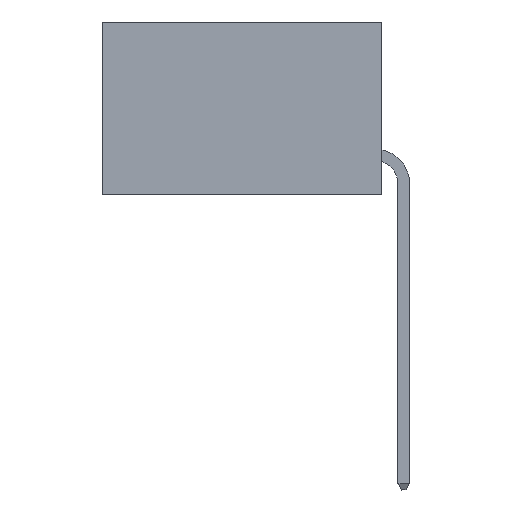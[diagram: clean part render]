
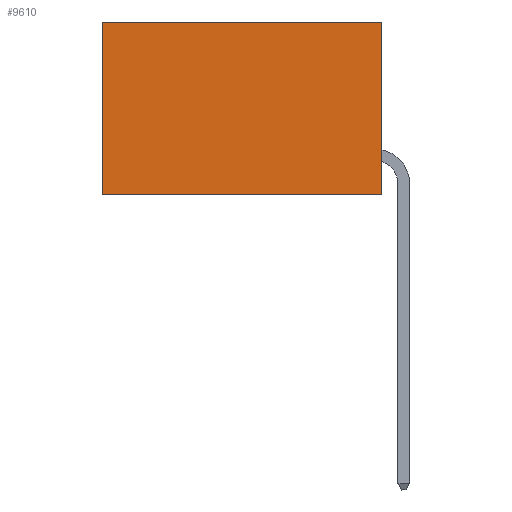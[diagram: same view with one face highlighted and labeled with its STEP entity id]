
A CAD part, left-side view. The second image highlights one B-rep face of the part: STEP entity #9610.
In plain terms, the highlighted planar face has unit normal (-1, 0, 0).
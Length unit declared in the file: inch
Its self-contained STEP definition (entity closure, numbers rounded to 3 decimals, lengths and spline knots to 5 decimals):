
#6 = EDGE_CURVE ( 'NONE', #14427, #11223, #9712, .T. ) ;
#198 = DIRECTION ( 'NONE',  ( 0., 0., -1. ) ) ;
#289 = EDGE_CURVE ( 'NONE', #11223, #3295, #1938, .T. ) ;
#1352 = VECTOR ( 'NONE', #15638, 39.37008 ) ;
#1938 = LINE ( 'NONE', #3981, #13541 ) ;
#2998 = CARTESIAN_POINT ( 'NONE',  ( 0.2875, 0., 0. ) ) ;
#3295 = VERTEX_POINT ( 'NONE', #11561 ) ;
#3981 = CARTESIAN_POINT ( 'NONE',  ( 0.2875, 0.6, 0. ) ) ;
#6026 = ORIENTED_EDGE ( 'NONE', *, *, #6596, .F. ) ;
#6596 = EDGE_CURVE ( 'NONE', #14427, #11262, #14353, .T. ) ;
#7561 = VECTOR ( 'NONE', #11308, 39.37008 ) ;
#7683 = DIRECTION ( 'NONE',  ( 1., 0., 0. ) ) ;
#8550 = AXIS2_PLACEMENT_3D ( 'NONE', #10078, #7683, #10244 ) ;
#9610 = ADVANCED_FACE ( 'NONE', ( #10826 ), #11335, .F. ) ;
#9712 = LINE ( 'NONE', #2998, #16153 ) ;
#9950 = ORIENTED_EDGE ( 'NONE', *, *, #6, .T. ) ;
#10078 = CARTESIAN_POINT ( 'NONE',  ( 0.2875, 0., 0. ) ) ;
#10244 = DIRECTION ( 'NONE',  ( 0., 0., -1. ) ) ;
#10633 = CARTESIAN_POINT ( 'NONE',  ( 0.2875, 0., 0. ) ) ;
#10785 = DIRECTION ( 'NONE',  ( 0., 1., 0. ) ) ;
#10826 = FACE_OUTER_BOUND ( 'NONE', #16523, .T. ) ;
#11223 = VERTEX_POINT ( 'NONE', #13755 ) ;
#11262 = VERTEX_POINT ( 'NONE', #15258 ) ;
#11308 = DIRECTION ( 'NONE',  ( 0., 0., -1. ) ) ;
#11335 = PLANE ( 'NONE',  #8550 ) ;
#11391 = ORIENTED_EDGE ( 'NONE', *, *, #289, .T. ) ;
#11561 = CARTESIAN_POINT ( 'NONE',  ( 0.2875, 0.6, -0.37 ) ) ;
#12797 = EDGE_CURVE ( 'NONE', #11262, #3295, #12909, .T. ) ;
#12909 = LINE ( 'NONE', #15476, #1352 ) ;
#13541 = VECTOR ( 'NONE', #198, 39.37008 ) ;
#13755 = CARTESIAN_POINT ( 'NONE',  ( 0.2875, 0.6, 0. ) ) ;
#14353 = LINE ( 'NONE', #15233, #7561 ) ;
#14427 = VERTEX_POINT ( 'NONE', #10633 ) ;
#14947 = ORIENTED_EDGE ( 'NONE', *, *, #12797, .F. ) ;
#15233 = CARTESIAN_POINT ( 'NONE',  ( 0.2875, 0., 0. ) ) ;
#15258 = CARTESIAN_POINT ( 'NONE',  ( 0.2875, 0., -0.37 ) ) ;
#15476 = CARTESIAN_POINT ( 'NONE',  ( 0.2875, 0., -0.37 ) ) ;
#15638 = DIRECTION ( 'NONE',  ( 0., 1., 0. ) ) ;
#16153 = VECTOR ( 'NONE', #10785, 39.37008 ) ;
#16523 = EDGE_LOOP ( 'NONE', ( #11391, #14947, #6026, #9950 ) ) ;
